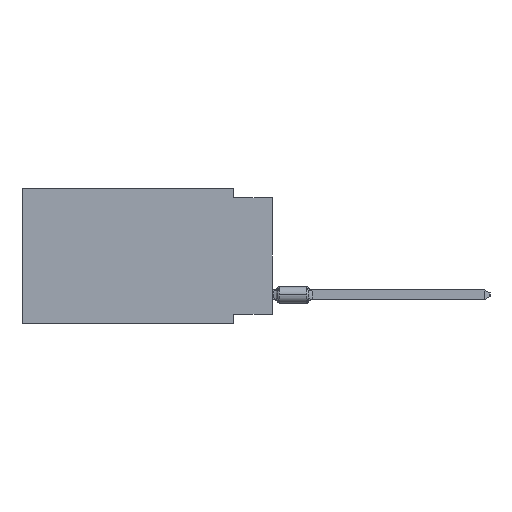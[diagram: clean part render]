
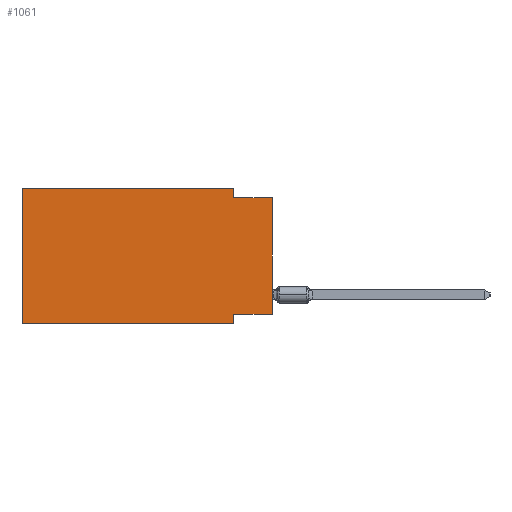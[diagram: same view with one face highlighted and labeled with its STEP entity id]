
A CAD part, left-side view. The second image highlights one B-rep face of the part: STEP entity #1061.
In plain terms, the highlighted planar face has unit normal (-1, 0, 0).
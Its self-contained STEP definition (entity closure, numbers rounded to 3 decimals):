
#335 = EDGE_CURVE ( 'NONE', #28792, #1020, #12706, .T. ) ;
#851 = VECTOR ( 'NONE', #17974, 1000. ) ;
#1020 = VERTEX_POINT ( 'NONE', #10224 ) ;
#1061 = ADVANCED_FACE ( 'NONE', ( #14709 ), #7450, .F. ) ;
#1758 = CARTESIAN_POINT ( 'NONE',  ( 0., 16.383, 0. ) ) ;
#2506 = CARTESIAN_POINT ( 'NONE',  ( 0., 0., -0.635 ) ) ;
#2779 = ORIENTED_EDGE ( 'NONE', *, *, #24478, .T. ) ;
#2829 = DIRECTION ( 'NONE',  ( 1., 0., 0. ) ) ;
#3440 = AXIS2_PLACEMENT_3D ( 'NONE', #12381, #2829, #28407 ) ;
#3768 = VECTOR ( 'NONE', #7578, 1000. ) ;
#5019 = LINE ( 'NONE', #12418, #26257 ) ;
#5226 = ORIENTED_EDGE ( 'NONE', *, *, #10710, .F. ) ;
#5445 = LINE ( 'NONE', #17023, #27695 ) ;
#5463 = VERTEX_POINT ( 'NONE', #19920 ) ;
#5908 = ORIENTED_EDGE ( 'NONE', *, *, #10788, .T. ) ;
#6596 = CARTESIAN_POINT ( 'NONE',  ( 0., 2.54, 0. ) ) ;
#6640 = ORIENTED_EDGE ( 'NONE', *, *, #14125, .F. ) ;
#7270 = LINE ( 'NONE', #28698, #3768 ) ;
#7296 = EDGE_CURVE ( 'NONE', #26827, #7548, #5019, .T. ) ;
#7350 = LINE ( 'NONE', #12118, #19803 ) ;
#7450 = PLANE ( 'NONE',  #3440 ) ;
#7548 = VERTEX_POINT ( 'NONE', #1758 ) ;
#7578 = DIRECTION ( 'NONE',  ( 0., -1., 0. ) ) ;
#8196 = VERTEX_POINT ( 'NONE', #26532 ) ;
#8821 = LINE ( 'NONE', #15629, #24492 ) ;
#10224 = CARTESIAN_POINT ( 'NONE',  ( 0., 2.54, -0.635 ) ) ;
#10710 = EDGE_CURVE ( 'NONE', #1020, #20178, #8821, .T. ) ;
#10788 = EDGE_CURVE ( 'NONE', #26827, #5463, #7270, .T. ) ;
#12118 = CARTESIAN_POINT ( 'NONE',  ( 0., 16.383, 0. ) ) ;
#12324 = CARTESIAN_POINT ( 'NONE',  ( 0., 0., -8.255 ) ) ;
#12381 = CARTESIAN_POINT ( 'NONE',  ( 0., 16.383, 0. ) ) ;
#12418 = CARTESIAN_POINT ( 'NONE',  ( 0., 16.383, 0. ) ) ;
#12706 = LINE ( 'NONE', #21949, #23225 ) ;
#12788 = LINE ( 'NONE', #24649, #17053 ) ;
#13593 = EDGE_CURVE ( 'NONE', #7548, #28792, #7350, .T. ) ;
#14125 = EDGE_CURVE ( 'NONE', #19129, #8196, #5445, .T. ) ;
#14190 = CARTESIAN_POINT ( 'NONE',  ( 0., 16.383, -8.89 ) ) ;
#14709 = FACE_OUTER_BOUND ( 'NONE', #25812, .T. ) ;
#15629 = CARTESIAN_POINT ( 'NONE',  ( 0., 0., -0.635 ) ) ;
#16873 = DIRECTION ( 'NONE',  ( 0., 1., 0. ) ) ;
#17023 = CARTESIAN_POINT ( 'NONE',  ( 0., 0., -8.255 ) ) ;
#17053 = VECTOR ( 'NONE', #19723, 1000. ) ;
#17974 = DIRECTION ( 'NONE',  ( 0., 0., 1. ) ) ;
#18002 = ORIENTED_EDGE ( 'NONE', *, *, #13593, .F. ) ;
#19071 = CARTESIAN_POINT ( 'NONE',  ( 0., 0., 0. ) ) ;
#19129 = VERTEX_POINT ( 'NONE', #12324 ) ;
#19490 = DIRECTION ( 'NONE',  ( 0., 0., -1. ) ) ;
#19723 = DIRECTION ( 'NONE',  ( 0., 0., -1. ) ) ;
#19803 = VECTOR ( 'NONE', #23379, 1000. ) ;
#19920 = CARTESIAN_POINT ( 'NONE',  ( 0., 2.54, -8.89 ) ) ;
#20178 = VERTEX_POINT ( 'NONE', #2506 ) ;
#20781 = ORIENTED_EDGE ( 'NONE', *, *, #7296, .F. ) ;
#20841 = DIRECTION ( 'NONE',  ( 0., -1., 0. ) ) ;
#21383 = LINE ( 'NONE', #19071, #851 ) ;
#21675 = DIRECTION ( 'NONE',  ( 0., 0., 1. ) ) ;
#21949 = CARTESIAN_POINT ( 'NONE',  ( 0., 2.54, 0. ) ) ;
#23225 = VECTOR ( 'NONE', #19490, 1000. ) ;
#23379 = DIRECTION ( 'NONE',  ( 0., -1., 0. ) ) ;
#24353 = ORIENTED_EDGE ( 'NONE', *, *, #335, .F. ) ;
#24478 = EDGE_CURVE ( 'NONE', #19129, #20178, #21383, .T. ) ;
#24492 = VECTOR ( 'NONE', #20841, 1000. ) ;
#24649 = CARTESIAN_POINT ( 'NONE',  ( 0., 2.54, -8.89 ) ) ;
#25812 = EDGE_LOOP ( 'NONE', ( #2779, #5226, #24353, #18002, #20781, #5908, #27088, #6640 ) ) ;
#26257 = VECTOR ( 'NONE', #21675, 1000. ) ;
#26532 = CARTESIAN_POINT ( 'NONE',  ( 0., 2.54, -8.255 ) ) ;
#26827 = VERTEX_POINT ( 'NONE', #14190 ) ;
#26949 = EDGE_CURVE ( 'NONE', #8196, #5463, #12788, .T. ) ;
#27088 = ORIENTED_EDGE ( 'NONE', *, *, #26949, .F. ) ;
#27695 = VECTOR ( 'NONE', #16873, 1000. ) ;
#28407 = DIRECTION ( 'NONE',  ( 0., 0., -1. ) ) ;
#28698 = CARTESIAN_POINT ( 'NONE',  ( 0., 16.383, -8.89 ) ) ;
#28792 = VERTEX_POINT ( 'NONE', #6596 ) ;
